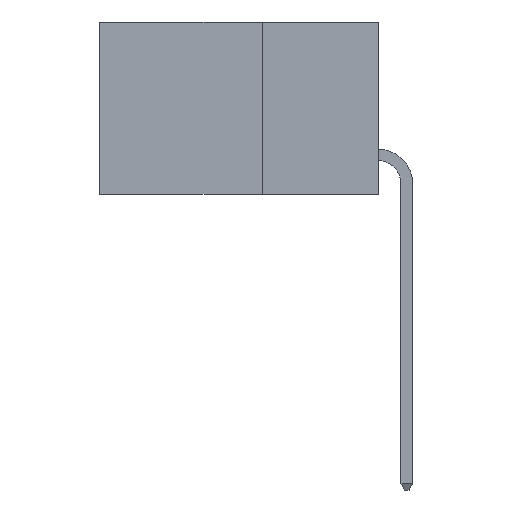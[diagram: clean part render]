
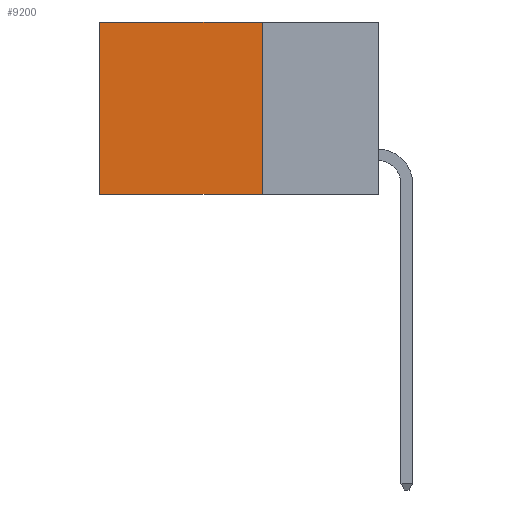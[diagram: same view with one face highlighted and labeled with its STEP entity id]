
A CAD part, left-side view. The second image highlights one B-rep face of the part: STEP entity #9200.
In plain terms, the highlighted planar face has unit normal (-1, 0, 0).
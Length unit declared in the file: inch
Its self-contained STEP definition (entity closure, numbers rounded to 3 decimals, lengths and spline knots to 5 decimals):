
#254 = EDGE_CURVE ( 'NONE', #15738, #5377, #16105, .T. ) ;
#271 = DIRECTION ( 'NONE',  ( 0., 0., -1. ) ) ;
#552 = ORIENTED_EDGE ( 'NONE', *, *, #254, .F. ) ;
#1795 = CARTESIAN_POINT ( 'NONE',  ( 0.2615, 0.25, -0.37 ) ) ;
#2125 = DIRECTION ( 'NONE',  ( 0., 0., -1. ) ) ;
#3792 = VECTOR ( 'NONE', #271, 39.37008 ) ;
#3965 = LINE ( 'NONE', #13326, #7114 ) ;
#3989 = DIRECTION ( 'NONE',  ( 0., 1., 0. ) ) ;
#4799 = CARTESIAN_POINT ( 'NONE',  ( 0.2615, 0.6, -0.37 ) ) ;
#5130 = VECTOR ( 'NONE', #2125, 39.37008 ) ;
#5377 = VERTEX_POINT ( 'NONE', #12235 ) ;
#5411 = EDGE_CURVE ( 'NONE', #10544, #12747, #10490, .T. ) ;
#5950 = PLANE ( 'NONE',  #13621 ) ;
#7114 = VECTOR ( 'NONE', #3989, 39.37008 ) ;
#7291 = DIRECTION ( 'NONE',  ( 1., 0., 0. ) ) ;
#7310 = LINE ( 'NONE', #11114, #10854 ) ;
#8396 = CARTESIAN_POINT ( 'NONE',  ( 0.2615, 0.6, -0.37 ) ) ;
#9200 = ADVANCED_FACE ( 'NONE', ( #15093 ), #5950, .F. ) ;
#10490 = LINE ( 'NONE', #8396, #3792 ) ;
#10544 = VERTEX_POINT ( 'NONE', #12903 ) ;
#10596 = EDGE_LOOP ( 'NONE', ( #13696, #10845, #552, #13798 ) ) ;
#10845 = ORIENTED_EDGE ( 'NONE', *, *, #12582, .F. ) ;
#10854 = VECTOR ( 'NONE', #12458, 39.37008 ) ;
#11114 = CARTESIAN_POINT ( 'NONE',  ( 0.2615, 0.25, -0.37 ) ) ;
#12235 = CARTESIAN_POINT ( 'NONE',  ( 0.2615, 0.25, -0.37 ) ) ;
#12350 = EDGE_CURVE ( 'NONE', #15738, #10544, #3965, .T. ) ;
#12458 = DIRECTION ( 'NONE',  ( 0., 1., 0. ) ) ;
#12582 = EDGE_CURVE ( 'NONE', #5377, #12747, #7310, .T. ) ;
#12747 = VERTEX_POINT ( 'NONE', #4799 ) ;
#12903 = CARTESIAN_POINT ( 'NONE',  ( 0.2615, 0.6, 0. ) ) ;
#13326 = CARTESIAN_POINT ( 'NONE',  ( 0.2615, 0.25, 0. ) ) ;
#13605 = CARTESIAN_POINT ( 'NONE',  ( 0.2615, 0.25, 0. ) ) ;
#13621 = AXIS2_PLACEMENT_3D ( 'NONE', #15226, #7291, #16541 ) ;
#13696 = ORIENTED_EDGE ( 'NONE', *, *, #5411, .T. ) ;
#13798 = ORIENTED_EDGE ( 'NONE', *, *, #12350, .T. ) ;
#15093 = FACE_OUTER_BOUND ( 'NONE', #10596, .T. ) ;
#15226 = CARTESIAN_POINT ( 'NONE',  ( 0.2615, 0.25, -0.37 ) ) ;
#15738 = VERTEX_POINT ( 'NONE', #13605 ) ;
#16105 = LINE ( 'NONE', #1795, #5130 ) ;
#16541 = DIRECTION ( 'NONE',  ( 0., 0., -1. ) ) ;
